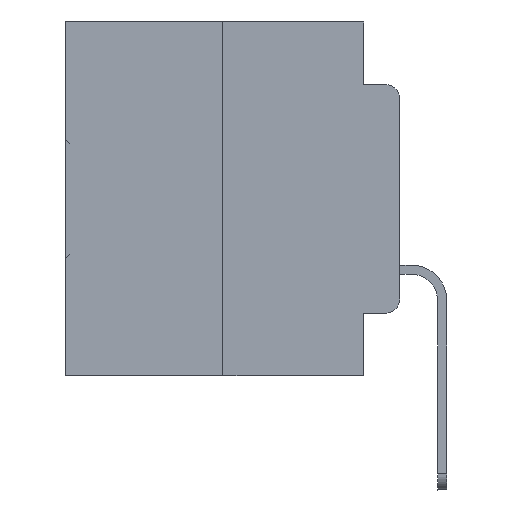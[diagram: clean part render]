
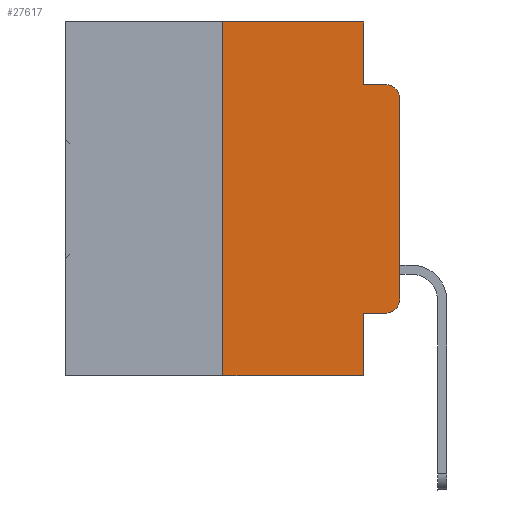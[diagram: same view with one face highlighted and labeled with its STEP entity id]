
A CAD part, left-side view. The second image highlights one B-rep face of the part: STEP entity #27617.
In plain terms, the highlighted planar face has unit normal (-1, 0, 0).
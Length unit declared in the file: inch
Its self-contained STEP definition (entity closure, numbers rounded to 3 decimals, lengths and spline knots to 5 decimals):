
#370 = VECTOR ( 'NONE', #10621, 39.37008 ) ;
#539 = CARTESIAN_POINT ( 'NONE',  ( 0., 0.02, -0.4115 ) ) ;
#595 = EDGE_CURVE ( 'NONE', #23728, #10331, #24667, .T. ) ;
#700 = LINE ( 'NONE', #27709, #20959 ) ;
#929 = CARTESIAN_POINT ( 'NONE',  ( 0., 0.051, -0.4115 ) ) ;
#985 = VECTOR ( 'NONE', #25281, 39.37008 ) ;
#2639 = DIRECTION ( 'NONE',  ( 0., 0., 1. ) ) ;
#2645 = CARTESIAN_POINT ( 'NONE',  ( 0., 0., -0.1085 ) ) ;
#2814 = VECTOR ( 'NONE', #24527, 39.37008 ) ;
#3161 = FACE_OUTER_BOUND ( 'NONE', #22219, .T. ) ;
#3269 = CARTESIAN_POINT ( 'NONE',  ( 0., 0.25, 0. ) ) ;
#3463 = AXIS2_PLACEMENT_3D ( 'NONE', #3684, #16663, #18320 ) ;
#3498 = CARTESIAN_POINT ( 'NONE',  ( 0., 0.051, -0.5 ) ) ;
#3684 = CARTESIAN_POINT ( 'NONE',  ( 0., 0.02, -0.3915 ) ) ;
#3736 = LINE ( 'NONE', #13067, #985 ) ;
#4357 = CARTESIAN_POINT ( 'NONE',  ( 0., 0.25, 0. ) ) ;
#4436 = ORIENTED_EDGE ( 'NONE', *, *, #19141, .T. ) ;
#4518 = CARTESIAN_POINT ( 'NONE',  ( 0., 0.473, -0.5 ) ) ;
#5208 = VERTEX_POINT ( 'NONE', #13800 ) ;
#5503 = VECTOR ( 'NONE', #9834, 39.37008 ) ;
#5549 = VERTEX_POINT ( 'NONE', #15859 ) ;
#5722 = CARTESIAN_POINT ( 'NONE',  ( 0., 0.02, -0.0885 ) ) ;
#7113 = ORIENTED_EDGE ( 'NONE', *, *, #28519, .F. ) ;
#7460 = CARTESIAN_POINT ( 'NONE',  ( 0., 0., -0.3915 ) ) ;
#7593 = CARTESIAN_POINT ( 'NONE',  ( 0., 0.02, -0.1085 ) ) ;
#8260 = DIRECTION ( 'NONE',  ( 0., -1., 0. ) ) ;
#9376 = EDGE_CURVE ( 'NONE', #21225, #9574, #14257, .T. ) ;
#9574 = VERTEX_POINT ( 'NONE', #5722 ) ;
#9834 = DIRECTION ( 'NONE',  ( 0., 0., 1. ) ) ;
#10141 = CIRCLE ( 'NONE', #3463, 0.02 ) ;
#10331 = VERTEX_POINT ( 'NONE', #4357 ) ;
#10621 = DIRECTION ( 'NONE',  ( 0., -1., 0. ) ) ;
#11686 = LINE ( 'NONE', #21479, #2814 ) ;
#12661 = VECTOR ( 'NONE', #28071, 39.37008 ) ;
#12963 = DIRECTION ( 'NONE',  ( 0., 0., -1. ) ) ;
#13067 = CARTESIAN_POINT ( 'NONE',  ( 0., 0.051, 0. ) ) ;
#13121 = DIRECTION ( 'NONE',  ( 1., 0., 0. ) ) ;
#13522 = EDGE_CURVE ( 'NONE', #19627, #9574, #17677, .T. ) ;
#13800 = CARTESIAN_POINT ( 'NONE',  ( 0., 0.051, -0.4115 ) ) ;
#14057 = AXIS2_PLACEMENT_3D ( 'NONE', #15540, #13121, #12963 ) ;
#14257 = LINE ( 'NONE', #24071, #370 ) ;
#14576 = ORIENTED_EDGE ( 'NONE', *, *, #25013, .F. ) ;
#15150 = ORIENTED_EDGE ( 'NONE', *, *, #13522, .T. ) ;
#15540 = CARTESIAN_POINT ( 'NONE',  ( 0., 0.473, 0. ) ) ;
#15859 = CARTESIAN_POINT ( 'NONE',  ( 0., 0.051, 0. ) ) ;
#16131 = ORIENTED_EDGE ( 'NONE', *, *, #30921, .T. ) ;
#16663 = DIRECTION ( 'NONE',  ( -1., 0., 0. ) ) ;
#17171 = ORIENTED_EDGE ( 'NONE', *, *, #22086, .T. ) ;
#17627 = PLANE ( 'NONE',  #14057 ) ;
#17636 = ORIENTED_EDGE ( 'NONE', *, *, #23027, .F. ) ;
#17677 = CIRCLE ( 'NONE', #22282, 0.02 ) ;
#18271 = LINE ( 'NONE', #929, #12661 ) ;
#18277 = ORIENTED_EDGE ( 'NONE', *, *, #595, .F. ) ;
#18320 = DIRECTION ( 'NONE',  ( 0., 0., -1. ) ) ;
#19141 = EDGE_CURVE ( 'NONE', #23728, #29600, #20056, .T. ) ;
#19326 = EDGE_CURVE ( 'NONE', #5208, #30371, #18271, .T. ) ;
#19627 = VERTEX_POINT ( 'NONE', #2645 ) ;
#19730 = DIRECTION ( 'NONE',  ( 0., -1., 0. ) ) ;
#19971 = DIRECTION ( 'NONE',  ( 0., 0., -1. ) ) ;
#20056 = LINE ( 'NONE', #4518, #22405 ) ;
#20959 = VECTOR ( 'NONE', #8260, 39.37008 ) ;
#21225 = VERTEX_POINT ( 'NONE', #24839 ) ;
#21479 = CARTESIAN_POINT ( 'NONE',  ( 0., 0.051, 0. ) ) ;
#21893 = LINE ( 'NONE', #26860, #5503 ) ;
#22086 = EDGE_CURVE ( 'NONE', #26246, #19627, #21893, .T. ) ;
#22167 = CARTESIAN_POINT ( 'NONE',  ( 0., 0.25, -0.5 ) ) ;
#22219 = EDGE_LOOP ( 'NONE', ( #17171, #15150, #24374, #7113, #17636, #18277, #4436, #14576, #29872, #16131 ) ) ;
#22282 = AXIS2_PLACEMENT_3D ( 'NONE', #7593, #30060, #19971 ) ;
#22405 = VECTOR ( 'NONE', #19730, 39.37008 ) ;
#23027 = EDGE_CURVE ( 'NONE', #10331, #5549, #700, .T. ) ;
#23728 = VERTEX_POINT ( 'NONE', #22167 ) ;
#24071 = CARTESIAN_POINT ( 'NONE',  ( 0., 0.051, -0.0885 ) ) ;
#24374 = ORIENTED_EDGE ( 'NONE', *, *, #9376, .F. ) ;
#24527 = DIRECTION ( 'NONE',  ( 0., 0., -1. ) ) ;
#24667 = LINE ( 'NONE', #3269, #27323 ) ;
#24839 = CARTESIAN_POINT ( 'NONE',  ( 0., 0.051, -0.0885 ) ) ;
#25013 = EDGE_CURVE ( 'NONE', #5208, #29600, #3736, .T. ) ;
#25281 = DIRECTION ( 'NONE',  ( 0., 0., -1. ) ) ;
#26246 = VERTEX_POINT ( 'NONE', #7460 ) ;
#26860 = CARTESIAN_POINT ( 'NONE',  ( 0., 0., 0. ) ) ;
#27323 = VECTOR ( 'NONE', #2639, 39.37008 ) ;
#27617 = ADVANCED_FACE ( 'NONE', ( #3161 ), #17627, .F. ) ;
#27709 = CARTESIAN_POINT ( 'NONE',  ( 0., 0.473, 0. ) ) ;
#28071 = DIRECTION ( 'NONE',  ( 0., -1., 0. ) ) ;
#28519 = EDGE_CURVE ( 'NONE', #5549, #21225, #11686, .T. ) ;
#29600 = VERTEX_POINT ( 'NONE', #3498 ) ;
#29872 = ORIENTED_EDGE ( 'NONE', *, *, #19326, .T. ) ;
#30060 = DIRECTION ( 'NONE',  ( -1., 0., 0. ) ) ;
#30371 = VERTEX_POINT ( 'NONE', #539 ) ;
#30921 = EDGE_CURVE ( 'NONE', #30371, #26246, #10141, .T. ) ;
